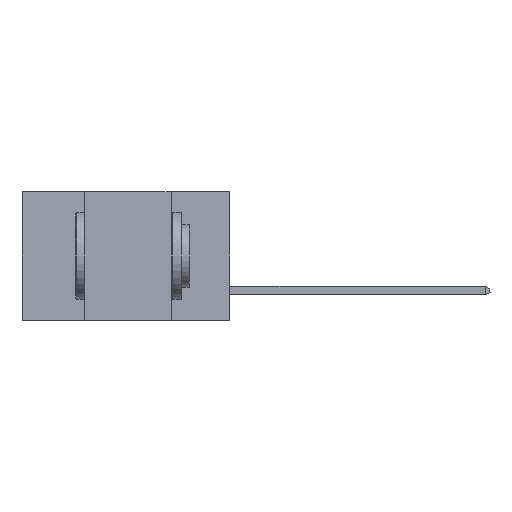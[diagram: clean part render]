
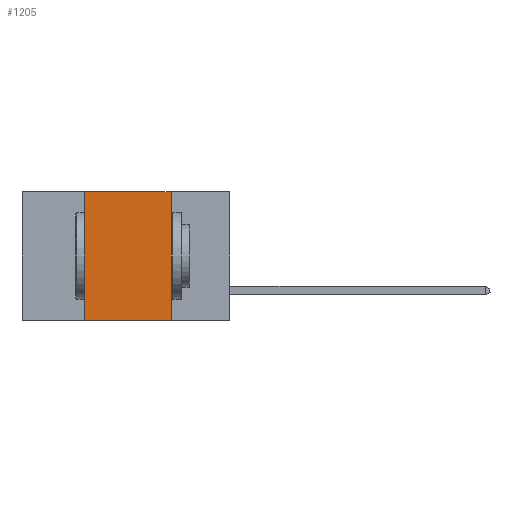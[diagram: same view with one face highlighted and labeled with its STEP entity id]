
A CAD part, left-side view. The second image highlights one B-rep face of the part: STEP entity #1205.
In plain terms, the highlighted planar face has unit normal (-1, 0, 0).
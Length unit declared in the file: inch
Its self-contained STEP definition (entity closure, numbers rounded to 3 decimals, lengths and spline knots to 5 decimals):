
#200 = ORIENTED_EDGE ( 'NONE', *, *, #19914, .F. ) ;
#768 = VECTOR ( 'NONE', #5900, 39.37008 ) ;
#1205 = ADVANCED_FACE ( 'NONE', ( #8975 ), #18533, .F. ) ;
#2201 = CARTESIAN_POINT ( 'NONE',  ( 0., 0.17, 0. ) ) ;
#2463 = VECTOR ( 'NONE', #10201, 39.37008 ) ;
#2755 = DIRECTION ( 'NONE',  ( 0., 0., -1. ) ) ;
#2998 = DIRECTION ( 'NONE',  ( 1., 0., 0. ) ) ;
#3397 = CARTESIAN_POINT ( 'NONE',  ( 0., 0.17, 0. ) ) ;
#4017 = VERTEX_POINT ( 'NONE', #10536 ) ;
#5479 = CARTESIAN_POINT ( 'NONE',  ( 0., 0.6, -0.37 ) ) ;
#5857 = LINE ( 'NONE', #11196, #768 ) ;
#5900 = DIRECTION ( 'NONE',  ( 0., -1., 0. ) ) ;
#6286 = EDGE_CURVE ( 'NONE', #12086, #14036, #5857, .T. ) ;
#6589 = VECTOR ( 'NONE', #21089, 39.37008 ) ;
#7282 = LINE ( 'NONE', #3397, #2463 ) ;
#8361 = VECTOR ( 'NONE', #19830, 39.37008 ) ;
#8975 = FACE_OUTER_BOUND ( 'NONE', #19167, .T. ) ;
#10201 = DIRECTION ( 'NONE',  ( 0., 0., -1. ) ) ;
#10536 = CARTESIAN_POINT ( 'NONE',  ( 0., 0.17, -0.37 ) ) ;
#11196 = CARTESIAN_POINT ( 'NONE',  ( 0., 0.6, 0. ) ) ;
#11388 = ORIENTED_EDGE ( 'NONE', *, *, #6286, .F. ) ;
#12086 = VERTEX_POINT ( 'NONE', #16590 ) ;
#12337 = CARTESIAN_POINT ( 'NONE',  ( 0., 0.42, 0. ) ) ;
#12659 = CARTESIAN_POINT ( 'NONE',  ( 0., 0.42, -0.37 ) ) ;
#13176 = LINE ( 'NONE', #5479, #8361 ) ;
#14036 = VERTEX_POINT ( 'NONE', #2201 ) ;
#14066 = AXIS2_PLACEMENT_3D ( 'NONE', #20321, #2998, #2755 ) ;
#15280 = LINE ( 'NONE', #12337, #6589 ) ;
#15782 = ORIENTED_EDGE ( 'NONE', *, *, #19996, .F. ) ;
#16027 = EDGE_CURVE ( 'NONE', #21968, #4017, #13176, .T. ) ;
#16590 = CARTESIAN_POINT ( 'NONE',  ( 0., 0.42, 0. ) ) ;
#18533 = PLANE ( 'NONE',  #14066 ) ;
#18919 = ORIENTED_EDGE ( 'NONE', *, *, #16027, .T. ) ;
#19167 = EDGE_LOOP ( 'NONE', ( #200, #11388, #15782, #18919 ) ) ;
#19830 = DIRECTION ( 'NONE',  ( 0., -1., 0. ) ) ;
#19914 = EDGE_CURVE ( 'NONE', #14036, #4017, #7282, .T. ) ;
#19996 = EDGE_CURVE ( 'NONE', #21968, #12086, #15280, .T. ) ;
#20321 = CARTESIAN_POINT ( 'NONE',  ( 0., 0.6, 0. ) ) ;
#21089 = DIRECTION ( 'NONE',  ( 0., 0., 1. ) ) ;
#21968 = VERTEX_POINT ( 'NONE', #12659 ) ;
